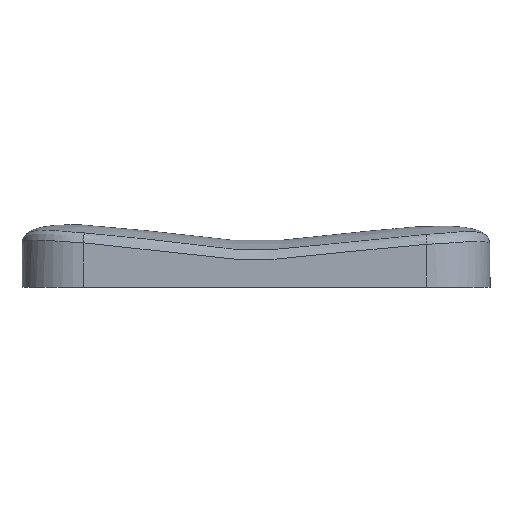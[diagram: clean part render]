
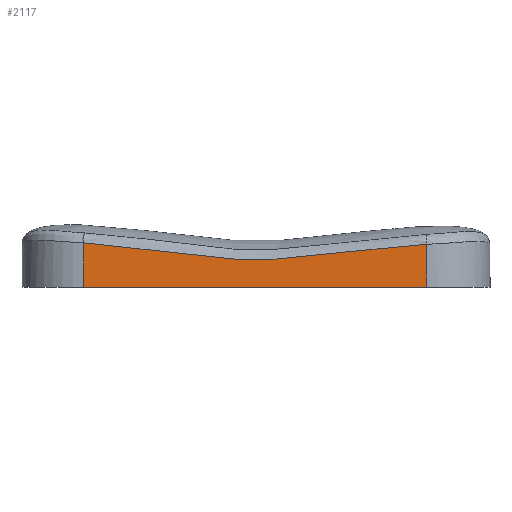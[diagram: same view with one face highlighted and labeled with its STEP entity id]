
A CAD part, left-side view. The second image highlights one B-rep face of the part: STEP entity #2117.
In plain terms, the highlighted planar face has unit normal (-1, 0, 0).
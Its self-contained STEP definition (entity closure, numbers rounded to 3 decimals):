
#6 = CARTESIAN_POINT ( 'NONE',  ( -18.555, -88.078, 12.581 ) ) ;
#14 = CARTESIAN_POINT ( 'NONE',  ( -18.555, 12.377, 13.014 ) ) ;
#16 = DIRECTION ( 'NONE',  ( 0., 1., 0. ) ) ;
#18 = DIRECTION ( 'NONE',  ( 1., 0., 0. ) ) ;
#21 = CARTESIAN_POINT ( 'NONE',  ( -18.555, 12.377, 5. ) ) ;
#31 = PLANE ( 'NONE',  #675 ) ;
#137 = B_SPLINE_CURVE_WITH_KNOTS ( 'NONE', 3,
 ( #1859, #2362, #1866, #1856, #1853, #1851, #1849, #1847, #1845, #1843, #1841, #1839, #1836, #1834, #1832, #1831, #1828, #1826, #1825, #1822, #1820, #1819, #1816, #1814, #1813, #1812, #1809, #1807, #1805, #1803 ),
 .UNSPECIFIED., .F., .F.,
 ( 4, 2, 2, 2, 2, 2, 2, 2, 2, 2, 2, 2, 2, 2, 4 ),
 ( 0., 0.006, 0.013, 0.025, 0.031, 0.038, 0.044, 0.05, 0.057, 0.063, 0.069, 0.076, 0.088, 0.094, 0.101 ),
 .UNSPECIFIED. ) ;
#366 = LINE ( 'NONE', #2530, #2447 ) ;
#528 = VERTEX_POINT ( 'NONE', #815 ) ;
#609 = CARTESIAN_POINT ( 'NONE',  ( -18.555, 12.377, 0. ) ) ;
#624 = ORIENTED_EDGE ( 'NONE', *, *, #1854, .T. ) ;
#636 = ORIENTED_EDGE ( 'NONE', *, *, #1818, .T. ) ;
#649 = VERTEX_POINT ( 'NONE', #749 ) ;
#674 = VERTEX_POINT ( 'NONE', #609 ) ;
#675 = AXIS2_PLACEMENT_3D ( 'NONE', #21, #18, #16 ) ;
#749 = CARTESIAN_POINT ( 'NONE',  ( -18.555, 12.377, 13.01 ) ) ;
#815 = CARTESIAN_POINT ( 'NONE',  ( -18.555, -88.078, 0. ) ) ;
#1074 = FACE_OUTER_BOUND ( 'NONE', #1830, .T. ) ;
#1289 = LINE ( 'NONE', #1862, #2650 ) ;
#1487 = VECTOR ( 'NONE', #1788, 1000. ) ;
#1499 = B_SPLINE_CURVE_WITH_KNOTS ( 'NONE', 3,
 ( #2055, #1857, #1794, #1792 ),
 .UNSPECIFIED., .F., .F.,
 ( 4, 4 ),
 ( 0., 0. ),
 .UNSPECIFIED. ) ;
#1762 = EDGE_CURVE ( 'NONE', #674, #528, #366, .T. ) ;
#1788 = DIRECTION ( 'NONE',  ( 0., 0., -1. ) ) ;
#1789 = CARTESIAN_POINT ( 'NONE',  ( -18.555, -88.078, 5. ) ) ;
#1792 = CARTESIAN_POINT ( 'NONE',  ( -18.555, 12.377, 13.01 ) ) ;
#1794 = CARTESIAN_POINT ( 'NONE',  ( -18.555, 12.377, 13.011 ) ) ;
#1803 = CARTESIAN_POINT ( 'NONE',  ( -18.555, 12.377, 13.014 ) ) ;
#1805 = CARTESIAN_POINT ( 'NONE',  ( -18.555, 10.267, 12.92 ) ) ;
#1807 = CARTESIAN_POINT ( 'NONE',  ( -18.555, 8.161, 12.764 ) ) ;
#1809 = CARTESIAN_POINT ( 'NONE',  ( -18.555, 3.955, 12.387 ) ) ;
#1812 = CARTESIAN_POINT ( 'NONE',  ( -18.555, 1.855, 12.165 ) ) ;
#1813 = CARTESIAN_POINT ( 'NONE',  ( -18.555, -4.437, 11.446 ) ) ;
#1814 = CARTESIAN_POINT ( 'NONE',  ( -18.555, -8.624, 10.893 ) ) ;
#1816 = CARTESIAN_POINT ( 'NONE',  ( -18.555, -14.904, 10.075 ) ) ;
#1818 = EDGE_CURVE ( 'NONE', #649, #674, #1289, .T. ) ;
#1819 = CARTESIAN_POINT ( 'NONE',  ( -18.555, -16.998, 9.803 ) ) ;
#1820 = CARTESIAN_POINT ( 'NONE',  ( -18.555, -21.188, 9.284 ) ) ;
#1822 = CARTESIAN_POINT ( 'NONE',  ( -18.555, -23.285, 9.036 ) ) ;
#1825 = CARTESIAN_POINT ( 'NONE',  ( -18.555, -27.484, 8.594 ) ) ;
#1826 = CARTESIAN_POINT ( 'NONE',  ( -18.555, -29.589, 8.4 ) ) ;
#1828 = CARTESIAN_POINT ( 'NONE',  ( -18.555, -33.791, 8.126 ) ) ;
#1830 = EDGE_LOOP ( 'NONE', ( #2358, #624, #636, #2115, #2285 ) ) ;
#1831 = CARTESIAN_POINT ( 'NONE',  ( -18.555, -35.889, 8.048 ) ) ;
#1832 = CARTESIAN_POINT ( 'NONE',  ( -18.555, -40.079, 8.042 ) ) ;
#1834 = CARTESIAN_POINT ( 'NONE',  ( -18.555, -42.171, 8.112 ) ) ;
#1836 = CARTESIAN_POINT ( 'NONE',  ( -18.555, -46.349, 8.363 ) ) ;
#1837 = EDGE_CURVE ( 'NONE', #2339, #2359, #137, .T. ) ;
#1839 = CARTESIAN_POINT ( 'NONE',  ( -18.555, -48.435, 8.54 ) ) ;
#1841 = CARTESIAN_POINT ( 'NONE',  ( -18.555, -52.606, 8.942 ) ) ;
#1843 = CARTESIAN_POINT ( 'NONE',  ( -18.555, -54.691, 9.168 ) ) ;
#1845 = CARTESIAN_POINT ( 'NONE',  ( -18.555, -58.858, 9.642 ) ) ;
#1847 = CARTESIAN_POINT ( 'NONE',  ( -18.555, -60.942, 9.889 ) ) ;
#1849 = CARTESIAN_POINT ( 'NONE',  ( -18.555, -67.192, 10.635 ) ) ;
#1851 = CARTESIAN_POINT ( 'NONE',  ( -18.555, -71.358, 11.138 ) ) ;
#1853 = CARTESIAN_POINT ( 'NONE',  ( -18.555, -77.617, 11.796 ) ) ;
#1854 = EDGE_CURVE ( 'NONE', #2359, #649, #1499, .T. ) ;
#1856 = CARTESIAN_POINT ( 'NONE',  ( -18.555, -79.705, 11.999 ) ) ;
#1857 = CARTESIAN_POINT ( 'NONE',  ( -18.555, 12.377, 13.013 ) ) ;
#1859 = CARTESIAN_POINT ( 'NONE',  ( -18.555, -88.078, 12.581 ) ) ;
#1861 = DIRECTION ( 'NONE',  ( 0., 0., -1. ) ) ;
#1862 = CARTESIAN_POINT ( 'NONE',  ( -18.555, 12.377, 5. ) ) ;
#1866 = CARTESIAN_POINT ( 'NONE',  ( -18.555, -83.886, 12.345 ) ) ;
#1867 = EDGE_CURVE ( 'NONE', #2339, #528, #1984, .T. ) ;
#1984 = LINE ( 'NONE', #1789, #1487 ) ;
#2055 = CARTESIAN_POINT ( 'NONE',  ( -18.555, 12.377, 13.014 ) ) ;
#2115 = ORIENTED_EDGE ( 'NONE', *, *, #1762, .T. ) ;
#2117 = ADVANCED_FACE ( 'NONE', ( #1074 ), #31, .F. ) ;
#2285 = ORIENTED_EDGE ( 'NONE', *, *, #1867, .F. ) ;
#2339 = VERTEX_POINT ( 'NONE', #6 ) ;
#2358 = ORIENTED_EDGE ( 'NONE', *, *, #1837, .T. ) ;
#2359 = VERTEX_POINT ( 'NONE', #14 ) ;
#2362 = CARTESIAN_POINT ( 'NONE',  ( -18.555, -85.98, 12.49 ) ) ;
#2447 = VECTOR ( 'NONE', #2535, 1000. ) ;
#2530 = CARTESIAN_POINT ( 'NONE',  ( -18.555, 12.377, 0. ) ) ;
#2535 = DIRECTION ( 'NONE',  ( 0., -1., 0. ) ) ;
#2650 = VECTOR ( 'NONE', #1861, 1000. ) ;
